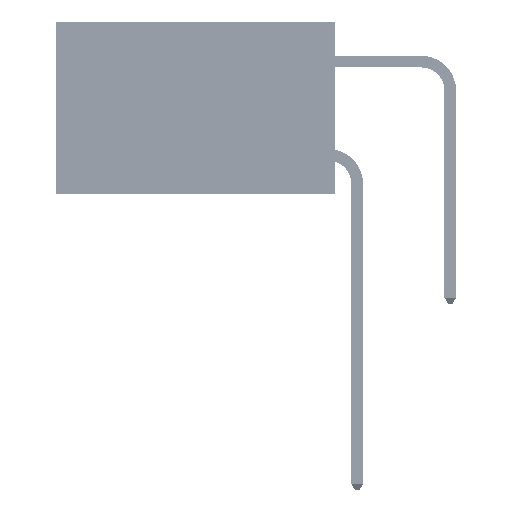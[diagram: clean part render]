
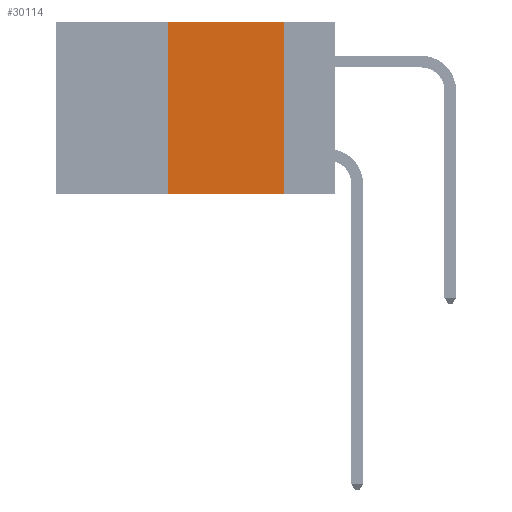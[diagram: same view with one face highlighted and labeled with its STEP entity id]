
A CAD part, left-side view. The second image highlights one B-rep face of the part: STEP entity #30114.
In plain terms, the highlighted planar face has unit normal (-1, 0, 0).
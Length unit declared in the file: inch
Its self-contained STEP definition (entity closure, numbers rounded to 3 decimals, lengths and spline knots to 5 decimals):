
#2509 = VECTOR ( 'NONE', #12471, 39.37008 ) ;
#3515 = LINE ( 'NONE', #36436, #6824 ) ;
#5808 = FACE_OUTER_BOUND ( 'NONE', #45574, .T. ) ;
#5949 = CARTESIAN_POINT ( 'NONE',  ( 0., 0.11, -0.37 ) ) ;
#6824 = VECTOR ( 'NONE', #18150, 39.37008 ) ;
#6924 = ORIENTED_EDGE ( 'NONE', *, *, #43197, .F. ) ;
#10225 = DIRECTION ( 'NONE',  ( 1., 0., 0. ) ) ;
#10534 = CARTESIAN_POINT ( 'NONE',  ( 0., 0.6, 0. ) ) ;
#10633 = VECTOR ( 'NONE', #39350, 39.37008 ) ;
#12471 = DIRECTION ( 'NONE',  ( 0., 0., -1. ) ) ;
#14292 = CARTESIAN_POINT ( 'NONE',  ( 0., 0.36, 0. ) ) ;
#14340 = ORIENTED_EDGE ( 'NONE', *, *, #16110, .T. ) ;
#15282 = VERTEX_POINT ( 'NONE', #5949 ) ;
#16110 = EDGE_CURVE ( 'NONE', #25594, #15282, #3515, .T. ) ;
#18150 = DIRECTION ( 'NONE',  ( 0., -1., 0. ) ) ;
#20971 = DIRECTION ( 'NONE',  ( 0., 0., -1. ) ) ;
#21077 = VERTEX_POINT ( 'NONE', #42168 ) ;
#23619 = CARTESIAN_POINT ( 'NONE',  ( 0., 0.36, -0.37 ) ) ;
#25209 = LINE ( 'NONE', #39039, #39584 ) ;
#25594 = VERTEX_POINT ( 'NONE', #23619 ) ;
#26356 = LINE ( 'NONE', #33718, #2509 ) ;
#29050 = VERTEX_POINT ( 'NONE', #43221 ) ;
#30114 = ADVANCED_FACE ( 'NONE', ( #5808 ), #31506, .F. ) ;
#30621 = LINE ( 'NONE', #14292, #10633 ) ;
#31506 = PLANE ( 'NONE',  #41777 ) ;
#32109 = DIRECTION ( 'NONE',  ( 0., -1., 0. ) ) ;
#33718 = CARTESIAN_POINT ( 'NONE',  ( 0., 0.11, 0. ) ) ;
#34515 = ORIENTED_EDGE ( 'NONE', *, *, #45297, .F. ) ;
#36436 = CARTESIAN_POINT ( 'NONE',  ( 0., 0.6, -0.37 ) ) ;
#39039 = CARTESIAN_POINT ( 'NONE',  ( 0., 0.6, 0. ) ) ;
#39350 = DIRECTION ( 'NONE',  ( 0., 0., 1. ) ) ;
#39584 = VECTOR ( 'NONE', #32109, 39.37008 ) ;
#40032 = ORIENTED_EDGE ( 'NONE', *, *, #44309, .F. ) ;
#41777 = AXIS2_PLACEMENT_3D ( 'NONE', #10534, #10225, #20971 ) ;
#42168 = CARTESIAN_POINT ( 'NONE',  ( 0., 0.11, 0. ) ) ;
#43197 = EDGE_CURVE ( 'NONE', #25594, #29050, #30621, .T. ) ;
#43221 = CARTESIAN_POINT ( 'NONE',  ( 0., 0.36, 0. ) ) ;
#44309 = EDGE_CURVE ( 'NONE', #29050, #21077, #25209, .T. ) ;
#45297 = EDGE_CURVE ( 'NONE', #21077, #15282, #26356, .T. ) ;
#45574 = EDGE_LOOP ( 'NONE', ( #34515, #40032, #6924, #14340 ) ) ;
